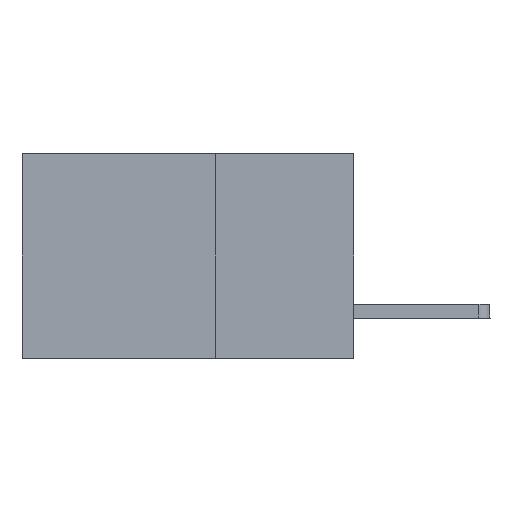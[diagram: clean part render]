
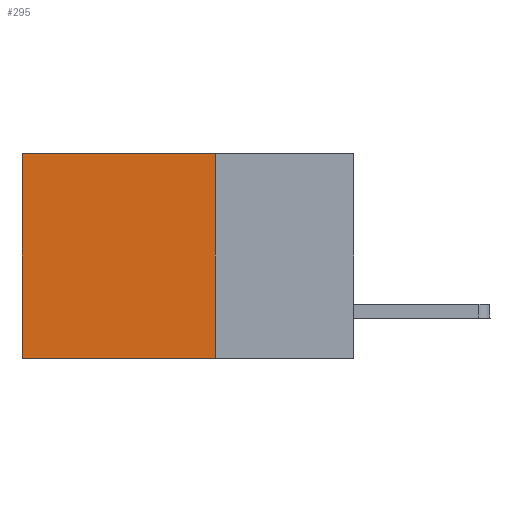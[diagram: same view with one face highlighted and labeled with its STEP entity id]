
A CAD part, left-side view. The second image highlights one B-rep face of the part: STEP entity #295.
In plain terms, the highlighted planar face has unit normal (-1, 0, 0).
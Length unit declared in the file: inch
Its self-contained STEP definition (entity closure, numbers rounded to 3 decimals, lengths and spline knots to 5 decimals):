
#295 = ADVANCED_FACE ( 'NONE', ( #6772 ), #1847, .F. ) ;
#1255 = DIRECTION ( 'NONE',  ( 0., 0., -1. ) ) ;
#1371 = VECTOR ( 'NONE', #7601, 39.37008 ) ;
#1847 = PLANE ( 'NONE',  #7535 ) ;
#2052 = VECTOR ( 'NONE', #13179, 39.37008 ) ;
#2491 = VERTEX_POINT ( 'NONE', #4320 ) ;
#2671 = CARTESIAN_POINT ( 'NONE',  ( 0.2875, 0.25, 0. ) ) ;
#4320 = CARTESIAN_POINT ( 'NONE',  ( 0.2875, 0.25, -0.37 ) ) ;
#4556 = VECTOR ( 'NONE', #9248, 39.37008 ) ;
#4780 = CARTESIAN_POINT ( 'NONE',  ( 0.2875, 0.6, 0. ) ) ;
#4841 = ORIENTED_EDGE ( 'NONE', *, *, #5623, .F. ) ;
#5526 = ORIENTED_EDGE ( 'NONE', *, *, #13941, .T. ) ;
#5623 = EDGE_CURVE ( 'NONE', #2491, #10410, #7680, .T. ) ;
#5664 = CARTESIAN_POINT ( 'NONE',  ( 0.2875, 0.25, 0. ) ) ;
#6212 = VERTEX_POINT ( 'NONE', #4780 ) ;
#6230 = DIRECTION ( 'NONE',  ( 1., 0., 0. ) ) ;
#6352 = DIRECTION ( 'NONE',  ( 0., 0., -1. ) ) ;
#6612 = VECTOR ( 'NONE', #1255, 39.37008 ) ;
#6772 = FACE_OUTER_BOUND ( 'NONE', #10102, .T. ) ;
#7440 = CARTESIAN_POINT ( 'NONE',  ( 0.2875, 0.6, -0.37 ) ) ;
#7535 = AXIS2_PLACEMENT_3D ( 'NONE', #8878, #6230, #6352 ) ;
#7601 = DIRECTION ( 'NONE',  ( 0., 1., 0. ) ) ;
#7646 = LINE ( 'NONE', #5664, #2052 ) ;
#7680 = LINE ( 'NONE', #8699, #1371 ) ;
#8699 = CARTESIAN_POINT ( 'NONE',  ( 0.2875, 0.25, -0.37 ) ) ;
#8878 = CARTESIAN_POINT ( 'NONE',  ( 0.2875, 0.25, 0. ) ) ;
#9031 = CARTESIAN_POINT ( 'NONE',  ( 0.2875, 0.6, 0. ) ) ;
#9248 = DIRECTION ( 'NONE',  ( 0., 0., -1. ) ) ;
#10102 = EDGE_LOOP ( 'NONE', ( #12725, #4841, #10596, #5526 ) ) ;
#10410 = VERTEX_POINT ( 'NONE', #7440 ) ;
#10596 = ORIENTED_EDGE ( 'NONE', *, *, #14164, .F. ) ;
#11306 = VERTEX_POINT ( 'NONE', #11321 ) ;
#11321 = CARTESIAN_POINT ( 'NONE',  ( 0.2875, 0.25, 0. ) ) ;
#12725 = ORIENTED_EDGE ( 'NONE', *, *, #14026, .T. ) ;
#13140 = LINE ( 'NONE', #2671, #4556 ) ;
#13179 = DIRECTION ( 'NONE',  ( 0., 1., 0. ) ) ;
#13314 = LINE ( 'NONE', #9031, #6612 ) ;
#13941 = EDGE_CURVE ( 'NONE', #11306, #6212, #7646, .T. ) ;
#14026 = EDGE_CURVE ( 'NONE', #6212, #10410, #13314, .T. ) ;
#14164 = EDGE_CURVE ( 'NONE', #11306, #2491, #13140, .T. ) ;
